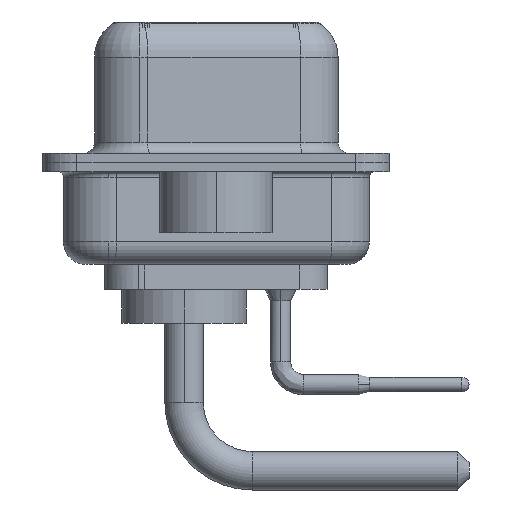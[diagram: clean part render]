
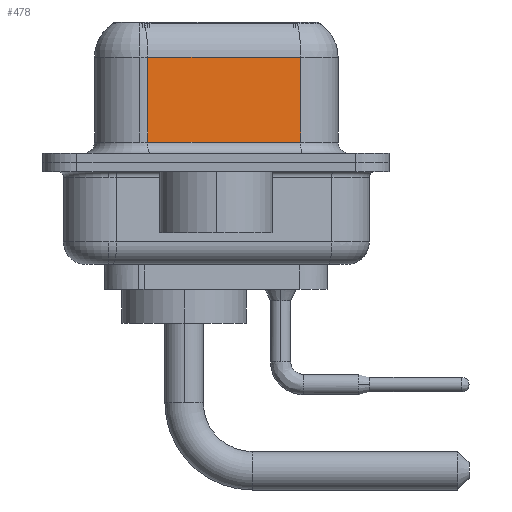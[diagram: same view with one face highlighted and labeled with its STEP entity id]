
A CAD part, left-side view. The second image highlights one B-rep face of the part: STEP entity #478.
In plain terms, the highlighted planar face has unit normal (-0.985, -0.174, 0).
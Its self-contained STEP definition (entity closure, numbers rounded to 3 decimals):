
#51 = CARTESIAN_POINT ( 'NONE',  ( 4.43, 3.028, 6.4 ) ) ;
#478 = ADVANCED_FACE ( 'NONE', ( #10100 ), #2898, .F. ) ;
#837 = CARTESIAN_POINT ( 'NONE',  ( 5.621, -3.722, 4.65 ) ) ;
#1716 = VECTOR ( 'NONE', #17168, 1000. ) ;
#2257 = VERTEX_POINT ( 'NONE', #11776 ) ;
#2898 = PLANE ( 'NONE',  #13950 ) ;
#2910 = LINE ( 'NONE', #19165, #1716 ) ;
#3047 = ORIENTED_EDGE ( 'NONE', *, *, #15410, .T. ) ;
#4397 = EDGE_CURVE ( 'NONE', #20818, #11829, #2910, .T. ) ;
#5056 = LINE ( 'NONE', #11616, #11091 ) ;
#5932 = CARTESIAN_POINT ( 'NONE',  ( 5.621, -3.722, 6.4 ) ) ;
#6776 = EDGE_CURVE ( 'NONE', #20818, #2257, #19199, .T. ) ;
#7894 = ORIENTED_EDGE ( 'NONE', *, *, #6776, .F. ) ;
#8660 = EDGE_CURVE ( 'NONE', #9130, #2257, #5056, .T. ) ;
#9009 = DIRECTION ( 'NONE',  ( -0.174, 0.985, 0. ) ) ;
#9130 = VERTEX_POINT ( 'NONE', #13088 ) ;
#9800 = ORIENTED_EDGE ( 'NONE', *, *, #4397, .T. ) ;
#10100 = FACE_OUTER_BOUND ( 'NONE', #14645, .T. ) ;
#11091 = VECTOR ( 'NONE', #14918, 1000. ) ;
#11548 = DIRECTION ( 'NONE',  ( 0., 0., -1. ) ) ;
#11616 = CARTESIAN_POINT ( 'NONE',  ( 5.621, -3.722, 0.9 ) ) ;
#11776 = CARTESIAN_POINT ( 'NONE',  ( 5.621, -3.722, 0.9 ) ) ;
#11829 = VERTEX_POINT ( 'NONE', #16188 ) ;
#12599 = DIRECTION ( 'NONE',  ( 0., 0., -1. ) ) ;
#13019 = ORIENTED_EDGE ( 'NONE', *, *, #8660, .T. ) ;
#13088 = CARTESIAN_POINT ( 'NONE',  ( 4.43, 3.028, 0.9 ) ) ;
#13950 = AXIS2_PLACEMENT_3D ( 'NONE', #17155, #17461, #9009 ) ;
#14645 = EDGE_LOOP ( 'NONE', ( #7894, #9800, #3047, #13019 ) ) ;
#14918 = DIRECTION ( 'NONE',  ( 0.174, -0.985, 0. ) ) ;
#15410 = EDGE_CURVE ( 'NONE', #11829, #9130, #19221, .T. ) ;
#15836 = VECTOR ( 'NONE', #12599, 1000. ) ;
#16188 = CARTESIAN_POINT ( 'NONE',  ( 4.43, 3.028, 4.65 ) ) ;
#17155 = CARTESIAN_POINT ( 'NONE',  ( 5.621, -3.722, 6.4 ) ) ;
#17168 = DIRECTION ( 'NONE',  ( -0.174, 0.985, 0. ) ) ;
#17461 = DIRECTION ( 'NONE',  ( 0.985, 0.174, 0. ) ) ;
#18646 = VECTOR ( 'NONE', #11548, 1000. ) ;
#19165 = CARTESIAN_POINT ( 'NONE',  ( 5.621, -3.722, 4.65 ) ) ;
#19199 = LINE ( 'NONE', #5932, #15836 ) ;
#19221 = LINE ( 'NONE', #51, #18646 ) ;
#20818 = VERTEX_POINT ( 'NONE', #837 ) ;
